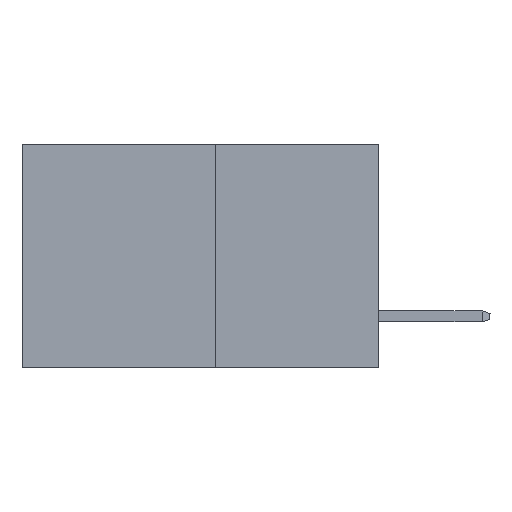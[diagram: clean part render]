
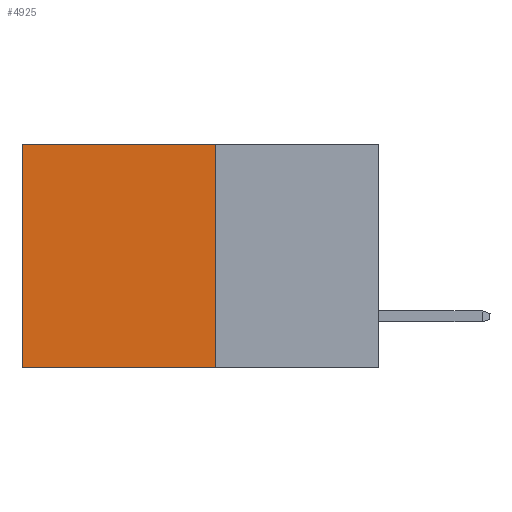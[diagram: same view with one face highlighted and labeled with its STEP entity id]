
A CAD part, left-side view. The second image highlights one B-rep face of the part: STEP entity #4925.
In plain terms, the highlighted planar face has unit normal (-1, 0, 0).
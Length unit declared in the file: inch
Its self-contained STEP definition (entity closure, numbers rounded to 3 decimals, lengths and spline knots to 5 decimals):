
#468 = CARTESIAN_POINT ( 'NONE',  ( 0.277, 0.27, -0.37 ) ) ;
#1088 = DIRECTION ( 'NONE',  ( 0., 0., -1. ) ) ;
#1304 = VERTEX_POINT ( 'NONE', #9729 ) ;
#1349 = VERTEX_POINT ( 'NONE', #2300 ) ;
#2300 = CARTESIAN_POINT ( 'NONE',  ( 0.277, 0.59, -0.37 ) ) ;
#2325 = ORIENTED_EDGE ( 'NONE', *, *, #6826, .T. ) ;
#2420 = DIRECTION ( 'NONE',  ( 0., 1., 0. ) ) ;
#2588 = DIRECTION ( 'NONE',  ( 1., 0., 0. ) ) ;
#2778 = ORIENTED_EDGE ( 'NONE', *, *, #5611, .F. ) ;
#2831 = PLANE ( 'NONE',  #9204 ) ;
#3017 = CARTESIAN_POINT ( 'NONE',  ( 0.277, 0.27, -0.37 ) ) ;
#3026 = DIRECTION ( 'NONE',  ( 0., 0., -1. ) ) ;
#3766 = FACE_OUTER_BOUND ( 'NONE', #7090, .T. ) ;
#3847 = CARTESIAN_POINT ( 'NONE',  ( 0.277, 0.27, 0. ) ) ;
#4284 = ORIENTED_EDGE ( 'NONE', *, *, #10953, .F. ) ;
#4718 = LINE ( 'NONE', #5835, #10608 ) ;
#4925 = ADVANCED_FACE ( 'NONE', ( #3766 ), #2831, .F. ) ;
#5176 = VECTOR ( 'NONE', #10974, 39.37008 ) ;
#5549 = VECTOR ( 'NONE', #11079, 39.37008 ) ;
#5611 = EDGE_CURVE ( 'NONE', #8544, #1349, #7497, .T. ) ;
#5835 = CARTESIAN_POINT ( 'NONE',  ( 0.277, 0.59, -0.37 ) ) ;
#6698 = LINE ( 'NONE', #11278, #8776 ) ;
#6826 = EDGE_CURVE ( 'NONE', #9044, #1304, #6698, .T. ) ;
#7041 = ORIENTED_EDGE ( 'NONE', *, *, #10274, .T. ) ;
#7090 = EDGE_LOOP ( 'NONE', ( #7041, #2778, #4284, #2325 ) ) ;
#7497 = LINE ( 'NONE', #3017, #5176 ) ;
#8544 = VERTEX_POINT ( 'NONE', #9372 ) ;
#8776 = VECTOR ( 'NONE', #2420, 39.37008 ) ;
#9044 = VERTEX_POINT ( 'NONE', #3847 ) ;
#9204 = AXIS2_PLACEMENT_3D ( 'NONE', #468, #2588, #3026 ) ;
#9372 = CARTESIAN_POINT ( 'NONE',  ( 0.277, 0.27, -0.37 ) ) ;
#9729 = CARTESIAN_POINT ( 'NONE',  ( 0.277, 0.59, 0. ) ) ;
#10181 = LINE ( 'NONE', #10233, #5549 ) ;
#10233 = CARTESIAN_POINT ( 'NONE',  ( 0.277, 0.27, -0.37 ) ) ;
#10274 = EDGE_CURVE ( 'NONE', #1304, #1349, #4718, .T. ) ;
#10608 = VECTOR ( 'NONE', #1088, 39.37008 ) ;
#10953 = EDGE_CURVE ( 'NONE', #9044, #8544, #10181, .T. ) ;
#10974 = DIRECTION ( 'NONE',  ( 0., 1., 0. ) ) ;
#11079 = DIRECTION ( 'NONE',  ( 0., 0., -1. ) ) ;
#11278 = CARTESIAN_POINT ( 'NONE',  ( 0.277, 0.27, 0. ) ) ;
